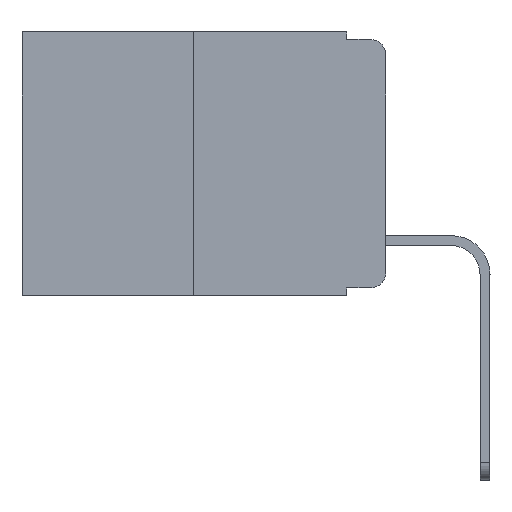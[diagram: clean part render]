
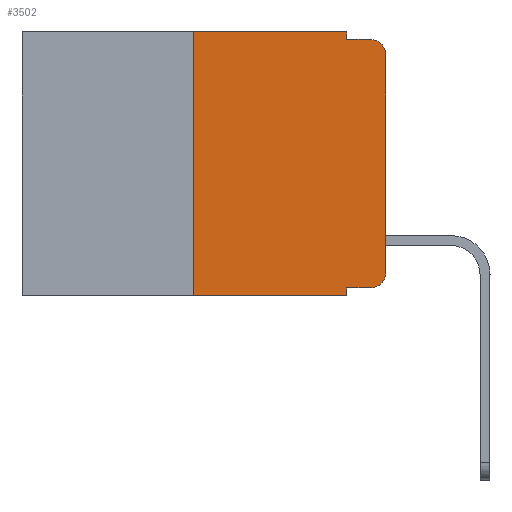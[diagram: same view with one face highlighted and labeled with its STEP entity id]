
A CAD part, left-side view. The second image highlights one B-rep face of the part: STEP entity #3502.
In plain terms, the highlighted planar face has unit normal (-1, 0, 0).
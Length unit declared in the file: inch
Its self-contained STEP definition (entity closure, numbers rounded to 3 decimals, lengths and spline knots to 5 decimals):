
#71 = CARTESIAN_POINT ( 'NONE',  ( 0., 0.25, -0.343 ) ) ;
#388 = DIRECTION ( 'NONE',  ( 1., 0., 0. ) ) ;
#389 = DIRECTION ( 'NONE',  ( 0., -1., 0. ) ) ;
#456 = LINE ( 'NONE', #1469, #9376 ) ;
#496 = EDGE_CURVE ( 'NONE', #10075, #4153, #2531, .T. ) ;
#540 = CARTESIAN_POINT ( 'NONE',  ( 0., 0.473, -0.343 ) ) ;
#558 = EDGE_CURVE ( 'NONE', #1230, #1220, #456, .T. ) ;
#638 = CARTESIAN_POINT ( 'NONE',  ( 0., 0.25, 0. ) ) ;
#834 = LINE ( 'NONE', #7663, #9161 ) ;
#917 = EDGE_LOOP ( 'NONE', ( #8125, #3342, #6658, #7147, #2972, #2181, #8014, #9963, #3522, #8328 ) ) ;
#1122 = PLANE ( 'NONE',  #3513 ) ;
#1157 = DIRECTION ( 'NONE',  ( 0., 0., -1. ) ) ;
#1160 = DIRECTION ( 'NONE',  ( 0., 0., -1. ) ) ;
#1220 = VERTEX_POINT ( 'NONE', #8817 ) ;
#1230 = VERTEX_POINT ( 'NONE', #4143 ) ;
#1410 = DIRECTION ( 'NONE',  ( 0., -1., 0. ) ) ;
#1469 = CARTESIAN_POINT ( 'NONE',  ( 0., 0.051, 0. ) ) ;
#1605 = CARTESIAN_POINT ( 'NONE',  ( 0., 0.02, -0.333 ) ) ;
#2011 = CARTESIAN_POINT ( 'NONE',  ( 0., 0.473, 0. ) ) ;
#2028 = AXIS2_PLACEMENT_3D ( 'NONE', #7834, #3138, #3965 ) ;
#2181 = ORIENTED_EDGE ( 'NONE', *, *, #496, .F. ) ;
#2248 = EDGE_CURVE ( 'NONE', #2485, #2636, #6185, .T. ) ;
#2485 = VERTEX_POINT ( 'NONE', #5971 ) ;
#2523 = CIRCLE ( 'NONE', #2028, 0.02 ) ;
#2531 = LINE ( 'NONE', #9306, #4388 ) ;
#2594 = FACE_OUTER_BOUND ( 'NONE', #917, .T. ) ;
#2636 = VERTEX_POINT ( 'NONE', #6312 ) ;
#2895 = EDGE_CURVE ( 'NONE', #2485, #4905, #10064, .T. ) ;
#2972 = ORIENTED_EDGE ( 'NONE', *, *, #8420, .F. ) ;
#3138 = DIRECTION ( 'NONE',  ( -1., 0., 0. ) ) ;
#3342 = ORIENTED_EDGE ( 'NONE', *, *, #7794, .T. ) ;
#3434 = CARTESIAN_POINT ( 'NONE',  ( 0., 0.02, -0.313 ) ) ;
#3436 = EDGE_CURVE ( 'NONE', #9739, #4809, #7280, .T. ) ;
#3452 = DIRECTION ( 'NONE',  ( 0., -1., 0. ) ) ;
#3470 = CARTESIAN_POINT ( 'NONE',  ( 0., 0., 0. ) ) ;
#3502 = ADVANCED_FACE ( 'NONE', ( #2594 ), #1122, .F. ) ;
#3513 = AXIS2_PLACEMENT_3D ( 'NONE', #2011, #388, #1157 ) ;
#3522 = ORIENTED_EDGE ( 'NONE', *, *, #2895, .T. ) ;
#3965 = DIRECTION ( 'NONE',  ( 0., 0., -1. ) ) ;
#4143 = CARTESIAN_POINT ( 'NONE',  ( 0., 0.051, 0. ) ) ;
#4153 = VERTEX_POINT ( 'NONE', #638 ) ;
#4221 = CARTESIAN_POINT ( 'NONE',  ( 0., 0., -0.313 ) ) ;
#4259 = DIRECTION ( 'NONE',  ( 0., 0., 1. ) ) ;
#4325 = CARTESIAN_POINT ( 'NONE',  ( 0., 0.051, -0.333 ) ) ;
#4388 = VECTOR ( 'NONE', #7792, 39.37008 ) ;
#4809 = VERTEX_POINT ( 'NONE', #6075 ) ;
#4905 = VERTEX_POINT ( 'NONE', #1605 ) ;
#5038 = DIRECTION ( 'NONE',  ( -1., 0., 0. ) ) ;
#5139 = EDGE_CURVE ( 'NONE', #4905, #9739, #8445, .T. ) ;
#5889 = EDGE_CURVE ( 'NONE', #1220, #6053, #834, .T. ) ;
#5971 = CARTESIAN_POINT ( 'NONE',  ( 0., 0.051, -0.333 ) ) ;
#6053 = VERTEX_POINT ( 'NONE', #7990 ) ;
#6060 = VECTOR ( 'NONE', #6560, 39.37008 ) ;
#6075 = CARTESIAN_POINT ( 'NONE',  ( 0., 0., -0.03 ) ) ;
#6185 = LINE ( 'NONE', #8937, #6060 ) ;
#6312 = CARTESIAN_POINT ( 'NONE',  ( 0., 0.051, -0.343 ) ) ;
#6560 = DIRECTION ( 'NONE',  ( 0., 0., -1. ) ) ;
#6580 = LINE ( 'NONE', #540, #9744 ) ;
#6658 = ORIENTED_EDGE ( 'NONE', *, *, #5889, .F. ) ;
#6965 = DIRECTION ( 'NONE',  ( 0., 0., -1. ) ) ;
#7147 = ORIENTED_EDGE ( 'NONE', *, *, #558, .F. ) ;
#7280 = LINE ( 'NONE', #3470, #7402 ) ;
#7402 = VECTOR ( 'NONE', #4259, 39.37008 ) ;
#7524 = EDGE_CURVE ( 'NONE', #10075, #2636, #6580, .T. ) ;
#7599 = AXIS2_PLACEMENT_3D ( 'NONE', #3434, #5038, #1160 ) ;
#7663 = CARTESIAN_POINT ( 'NONE',  ( 0., 0.051, -0.01 ) ) ;
#7792 = DIRECTION ( 'NONE',  ( 0., 0., 1. ) ) ;
#7794 = EDGE_CURVE ( 'NONE', #4809, #6053, #2523, .T. ) ;
#7834 = CARTESIAN_POINT ( 'NONE',  ( 0., 0.02, -0.03 ) ) ;
#7990 = CARTESIAN_POINT ( 'NONE',  ( 0., 0.02, -0.01 ) ) ;
#8014 = ORIENTED_EDGE ( 'NONE', *, *, #7524, .T. ) ;
#8125 = ORIENTED_EDGE ( 'NONE', *, *, #3436, .T. ) ;
#8150 = CARTESIAN_POINT ( 'NONE',  ( 0., 0.473, 0. ) ) ;
#8256 = VECTOR ( 'NONE', #389, 39.37008 ) ;
#8275 = DIRECTION ( 'NONE',  ( 0., -1., 0. ) ) ;
#8328 = ORIENTED_EDGE ( 'NONE', *, *, #5139, .T. ) ;
#8399 = LINE ( 'NONE', #8150, #9966 ) ;
#8420 = EDGE_CURVE ( 'NONE', #4153, #1230, #8399, .T. ) ;
#8445 = CIRCLE ( 'NONE', #7599, 0.02 ) ;
#8817 = CARTESIAN_POINT ( 'NONE',  ( 0., 0.051, -0.01 ) ) ;
#8937 = CARTESIAN_POINT ( 'NONE',  ( 0., 0.051, 0. ) ) ;
#9161 = VECTOR ( 'NONE', #1410, 39.37008 ) ;
#9306 = CARTESIAN_POINT ( 'NONE',  ( 0., 0.25, 0. ) ) ;
#9376 = VECTOR ( 'NONE', #6965, 39.37008 ) ;
#9739 = VERTEX_POINT ( 'NONE', #4221 ) ;
#9744 = VECTOR ( 'NONE', #8275, 39.37008 ) ;
#9963 = ORIENTED_EDGE ( 'NONE', *, *, #2248, .F. ) ;
#9966 = VECTOR ( 'NONE', #3452, 39.37008 ) ;
#10064 = LINE ( 'NONE', #4325, #8256 ) ;
#10075 = VERTEX_POINT ( 'NONE', #71 ) ;
